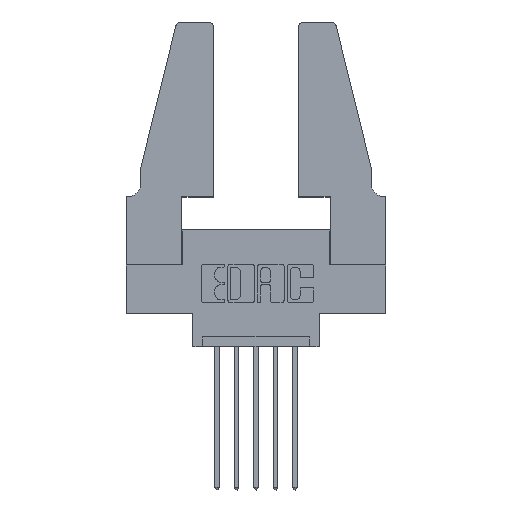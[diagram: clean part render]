
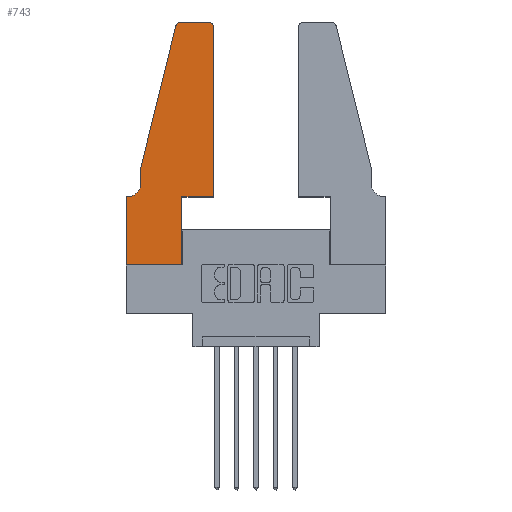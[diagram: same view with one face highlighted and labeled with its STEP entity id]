
A CAD part, top view. The second image highlights one B-rep face of the part: STEP entity #743.
In plain terms, the highlighted planar face has unit normal (0, 0, 1).
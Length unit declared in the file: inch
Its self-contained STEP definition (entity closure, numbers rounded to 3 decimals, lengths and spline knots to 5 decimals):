
#7 = DIRECTION ( 'NONE',  ( 1., 0., 0. ) ) ;
#203 = VERTEX_POINT ( 'NONE', #6214 ) ;
#216 = CARTESIAN_POINT ( 'NONE',  ( 0.2865, 0.35, 0.37 ) ) ;
#312 = DIRECTION ( 'NONE',  ( 1., 0., 0. ) ) ;
#334 = EDGE_LOOP ( 'NONE', ( #2292, #4751, #3733, #2357, #7839, #4655, #2414, #6066, #567, #1739, #4788, #6875 ) ) ;
#517 = CARTESIAN_POINT ( 'NONE',  ( 0.0055, 0.35, 0.37 ) ) ;
#567 = ORIENTED_EDGE ( 'NONE', *, *, #2380, .T. ) ;
#592 = DIRECTION ( 'NONE',  ( 0., 0., -1. ) ) ;
#601 = CARTESIAN_POINT ( 'NONE',  ( 0.4505, 1.22, 0.37 ) ) ;
#633 = LINE ( 'NONE', #6199, #2614 ) ;
#738 = CIRCLE ( 'NONE', #1042, 0.03 ) ;
#743 = ADVANCED_FACE ( 'NONE', ( #6801 ), #3767, .T. ) ;
#1042 = AXIS2_PLACEMENT_3D ( 'NONE', #3545, #4241, #7 ) ;
#1108 = DIRECTION ( 'NONE',  ( 0., 1., 0. ) ) ;
#1173 = AXIS2_PLACEMENT_3D ( 'NONE', #1253, #10689, #312 ) ;
#1231 = DIRECTION ( 'NONE',  ( -0.239, -0.971, 0. ) ) ;
#1253 = CARTESIAN_POINT ( 'NONE',  ( 0., 0.35, 0.37 ) ) ;
#1610 = VECTOR ( 'NONE', #5076, 39.37008 ) ;
#1705 = CARTESIAN_POINT ( 'NONE',  ( 0.0755, 0.35, 0.37 ) ) ;
#1739 = ORIENTED_EDGE ( 'NONE', *, *, #9288, .T. ) ;
#1924 = EDGE_CURVE ( 'NONE', #9228, #5542, #9740, .T. ) ;
#1988 = VERTEX_POINT ( 'NONE', #9572 ) ;
#2286 = VECTOR ( 'NONE', #7708, 39.37008 ) ;
#2292 = ORIENTED_EDGE ( 'NONE', *, *, #2950, .T. ) ;
#2357 = ORIENTED_EDGE ( 'NONE', *, *, #2575, .T. ) ;
#2380 = EDGE_CURVE ( 'NONE', #3880, #3214, #10127, .T. ) ;
#2414 = ORIENTED_EDGE ( 'NONE', *, *, #7174, .T. ) ;
#2477 = EDGE_CURVE ( 'NONE', #3547, #8673, #6950, .T. ) ;
#2575 = EDGE_CURVE ( 'NONE', #203, #6128, #633, .T. ) ;
#2614 = VECTOR ( 'NONE', #2763, 39.37008 ) ;
#2763 = DIRECTION ( 'NONE',  ( 0., -1., 0. ) ) ;
#2883 = LINE ( 'NONE', #3113, #7090 ) ;
#2950 = EDGE_CURVE ( 'NONE', #1988, #9228, #9703, .T. ) ;
#2989 = EDGE_CURVE ( 'NONE', #6009, #3880, #2883, .T. ) ;
#3113 = CARTESIAN_POINT ( 'NONE',  ( 0., 0., 0.37 ) ) ;
#3184 = DIRECTION ( 'NONE',  ( -1., 0., 0. ) ) ;
#3208 = CARTESIAN_POINT ( 'NONE',  ( 0.2865, 0., 0.37 ) ) ;
#3214 = VERTEX_POINT ( 'NONE', #216 ) ;
#3251 = EDGE_CURVE ( 'NONE', #5542, #203, #8749, .T. ) ;
#3307 = EDGE_CURVE ( 'NONE', #8673, #1988, #738, .T. ) ;
#3545 = CARTESIAN_POINT ( 'NONE',  ( 0.4205, 1.22, 0.37 ) ) ;
#3547 = VERTEX_POINT ( 'NONE', #6912 ) ;
#3733 = ORIENTED_EDGE ( 'NONE', *, *, #3251, .T. ) ;
#3767 = PLANE ( 'NONE',  #1173 ) ;
#3880 = VERTEX_POINT ( 'NONE', #3208 ) ;
#3924 = LINE ( 'NONE', #1705, #1610 ) ;
#4241 = DIRECTION ( 'NONE',  ( 0., 0., 1. ) ) ;
#4359 = VECTOR ( 'NONE', #1231, 39.37008 ) ;
#4543 = AXIS2_PLACEMENT_3D ( 'NONE', #10002, #8345, #9195 ) ;
#4655 = ORIENTED_EDGE ( 'NONE', *, *, #6267, .T. ) ;
#4751 = ORIENTED_EDGE ( 'NONE', *, *, #1924, .T. ) ;
#4788 = ORIENTED_EDGE ( 'NONE', *, *, #2477, .T. ) ;
#4805 = DIRECTION ( 'NONE',  ( -1., 0., 0. ) ) ;
#5076 = DIRECTION ( 'NONE',  ( -1., 0., 0. ) ) ;
#5152 = EDGE_CURVE ( 'NONE', #6128, #5638, #9128, .T. ) ;
#5351 = DIRECTION ( 'NONE',  ( 0., 1., 0. ) ) ;
#5437 = AXIS2_PLACEMENT_3D ( 'NONE', #10039, #592, #4805 ) ;
#5542 = VERTEX_POINT ( 'NONE', #8901 ) ;
#5638 = VERTEX_POINT ( 'NONE', #517 ) ;
#5766 = VECTOR ( 'NONE', #6994, 39.37008 ) ;
#5970 = VECTOR ( 'NONE', #3184, 39.37008 ) ;
#6009 = VERTEX_POINT ( 'NONE', #9070 ) ;
#6047 = VERTEX_POINT ( 'NONE', #6998 ) ;
#6066 = ORIENTED_EDGE ( 'NONE', *, *, #2989, .T. ) ;
#6128 = VERTEX_POINT ( 'NONE', #7295 ) ;
#6199 = CARTESIAN_POINT ( 'NONE',  ( 0.0755, 0.5, 0.37 ) ) ;
#6214 = CARTESIAN_POINT ( 'NONE',  ( 0.0755, 0.5, 0.37 ) ) ;
#6250 = CARTESIAN_POINT ( 'NONE',  ( 0.2865, 0.35, 0.37 ) ) ;
#6267 = EDGE_CURVE ( 'NONE', #5638, #6047, #3924, .T. ) ;
#6484 = LINE ( 'NONE', #10266, #2286 ) ;
#6801 = FACE_OUTER_BOUND ( 'NONE', #334, .T. ) ;
#6875 = ORIENTED_EDGE ( 'NONE', *, *, #3307, .T. ) ;
#6912 = CARTESIAN_POINT ( 'NONE',  ( 0.4505, 0.35, 0.37 ) ) ;
#6950 = LINE ( 'NONE', #7048, #10785 ) ;
#6994 = DIRECTION ( 'NONE',  ( 0., -1., 0. ) ) ;
#6998 = CARTESIAN_POINT ( 'NONE',  ( 0., 0.35, 0.37 ) ) ;
#7048 = CARTESIAN_POINT ( 'NONE',  ( 0.4505, 0.35, 0.37 ) ) ;
#7090 = VECTOR ( 'NONE', #7446, 39.37008 ) ;
#7155 = CARTESIAN_POINT ( 'NONE',  ( 0.2605, 1.25, 0.37 ) ) ;
#7174 = EDGE_CURVE ( 'NONE', #6047, #6009, #8032, .T. ) ;
#7213 = CARTESIAN_POINT ( 'NONE',  ( 0.284, 1.25, 0.37 ) ) ;
#7295 = CARTESIAN_POINT ( 'NONE',  ( 0.0755, 0.42, 0.37 ) ) ;
#7446 = DIRECTION ( 'NONE',  ( 1., 0., 0. ) ) ;
#7708 = DIRECTION ( 'NONE',  ( 1., 0., 0. ) ) ;
#7839 = ORIENTED_EDGE ( 'NONE', *, *, #5152, .T. ) ;
#8032 = LINE ( 'NONE', #8687, #5766 ) ;
#8345 = DIRECTION ( 'NONE',  ( 0., 0., 1. ) ) ;
#8673 = VERTEX_POINT ( 'NONE', #601 ) ;
#8687 = CARTESIAN_POINT ( 'NONE',  ( 0., 0., 0.37 ) ) ;
#8749 = LINE ( 'NONE', #10525, #4359 ) ;
#8901 = CARTESIAN_POINT ( 'NONE',  ( 0.25487, 1.22718, 0.37 ) ) ;
#9070 = CARTESIAN_POINT ( 'NONE',  ( 0., 0., 0.37 ) ) ;
#9128 = CIRCLE ( 'NONE', #5437, 0.07 ) ;
#9195 = DIRECTION ( 'NONE',  ( 1., 0., 0. ) ) ;
#9228 = VERTEX_POINT ( 'NONE', #7213 ) ;
#9288 = EDGE_CURVE ( 'NONE', #3214, #3547, #6484, .T. ) ;
#9572 = CARTESIAN_POINT ( 'NONE',  ( 0.4205, 1.25, 0.37 ) ) ;
#9703 = LINE ( 'NONE', #7155, #5970 ) ;
#9740 = CIRCLE ( 'NONE', #4543, 0.03 ) ;
#9859 = VECTOR ( 'NONE', #1108, 39.37008 ) ;
#10002 = CARTESIAN_POINT ( 'NONE',  ( 0.284, 1.22, 0.37 ) ) ;
#10039 = CARTESIAN_POINT ( 'NONE',  ( 0.0055, 0.42, 0.37 ) ) ;
#10127 = LINE ( 'NONE', #6250, #9859 ) ;
#10266 = CARTESIAN_POINT ( 'NONE',  ( 0.4505, 0.35, 0.37 ) ) ;
#10525 = CARTESIAN_POINT ( 'NONE',  ( 0.0755, 0.5, 0.37 ) ) ;
#10689 = DIRECTION ( 'NONE',  ( 0., 0., 1. ) ) ;
#10785 = VECTOR ( 'NONE', #5351, 39.37008 ) ;
